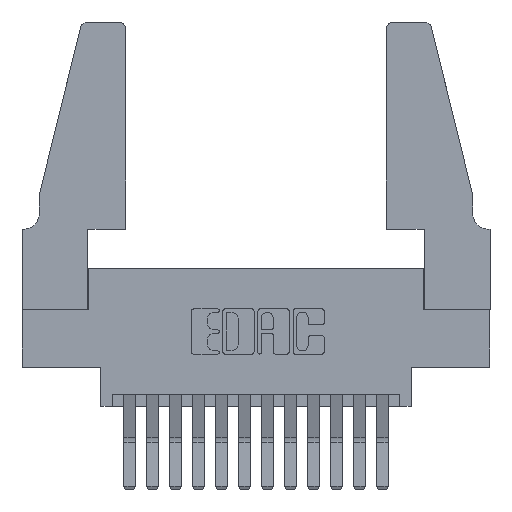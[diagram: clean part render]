
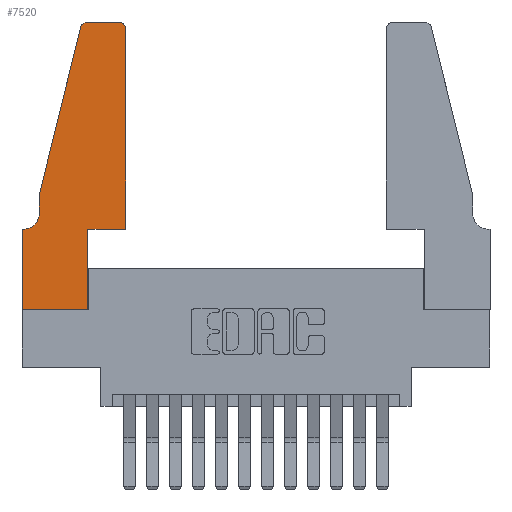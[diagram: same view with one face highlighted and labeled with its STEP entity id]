
A CAD part, top view. The second image highlights one B-rep face of the part: STEP entity #7520.
In plain terms, the highlighted planar face has unit normal (0, 0, 1).
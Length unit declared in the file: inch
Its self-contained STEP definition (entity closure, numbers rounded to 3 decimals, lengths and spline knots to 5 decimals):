
#479 = VECTOR ( 'NONE', #13768, 39.37008 ) ;
#505 = VERTEX_POINT ( 'NONE', #4299 ) ;
#840 = ORIENTED_EDGE ( 'NONE', *, *, #12736, .T. ) ;
#854 = ORIENTED_EDGE ( 'NONE', *, *, #15607, .T. ) ;
#908 = VERTEX_POINT ( 'NONE', #6339 ) ;
#961 = CARTESIAN_POINT ( 'NONE',  ( 0.0755, 0.35, 0.37 ) ) ;
#1022 = CIRCLE ( 'NONE', #14794, 0.07 ) ;
#1162 = CARTESIAN_POINT ( 'NONE',  ( 0.2865, 0.35, 0.37 ) ) ;
#1257 = VECTOR ( 'NONE', #4696, 39.37008 ) ;
#1304 = CARTESIAN_POINT ( 'NONE',  ( 0., 0., 0.37 ) ) ;
#1412 = ORIENTED_EDGE ( 'NONE', *, *, #11370, .T. ) ;
#1594 = CARTESIAN_POINT ( 'NONE',  ( 0.4505, 0.35, 0.37 ) ) ;
#1698 = EDGE_CURVE ( 'NONE', #505, #10028, #10328, .T. ) ;
#2288 = CARTESIAN_POINT ( 'NONE',  ( 0.4505, 0.35, 0.37 ) ) ;
#2584 = CARTESIAN_POINT ( 'NONE',  ( 0.4505, 0.35, 0.37 ) ) ;
#2768 = CARTESIAN_POINT ( 'NONE',  ( 0.0755, 0.5, 0.37 ) ) ;
#2805 = FACE_OUTER_BOUND ( 'NONE', #8059, .T. ) ;
#2942 = ORIENTED_EDGE ( 'NONE', *, *, #3870, .T. ) ;
#3148 = EDGE_CURVE ( 'NONE', #4799, #7429, #10499, .T. ) ;
#3247 = DIRECTION ( 'NONE',  ( 0., 1., 0. ) ) ;
#3351 = ORIENTED_EDGE ( 'NONE', *, *, #1698, .T. ) ;
#3458 = CIRCLE ( 'NONE', #11859, 0.03 ) ;
#3568 = LINE ( 'NONE', #2288, #15792 ) ;
#3857 = ORIENTED_EDGE ( 'NONE', *, *, #7246, .T. ) ;
#3870 = EDGE_CURVE ( 'NONE', #908, #11900, #13497, .T. ) ;
#4131 = LINE ( 'NONE', #1304, #12725 ) ;
#4299 = CARTESIAN_POINT ( 'NONE',  ( 0.0055, 0.35, 0.37 ) ) ;
#4397 = CARTESIAN_POINT ( 'NONE',  ( 0.0055, 0.42, 0.37 ) ) ;
#4409 = DIRECTION ( 'NONE',  ( -1., 0., 0. ) ) ;
#4422 = EDGE_CURVE ( 'NONE', #11900, #8486, #15194, .T. ) ;
#4696 = DIRECTION ( 'NONE',  ( -1., 0., 0. ) ) ;
#4799 = VERTEX_POINT ( 'NONE', #15461 ) ;
#4889 = PLANE ( 'NONE',  #12070 ) ;
#5091 = CARTESIAN_POINT ( 'NONE',  ( 0.284, 1.22, 0.37 ) ) ;
#5135 = DIRECTION ( 'NONE',  ( 0., 0., 1. ) ) ;
#5478 = ORIENTED_EDGE ( 'NONE', *, *, #8214, .T. ) ;
#5525 = CARTESIAN_POINT ( 'NONE',  ( 0.0755, 0.42, 0.37 ) ) ;
#5592 = CARTESIAN_POINT ( 'NONE',  ( 0.2605, 1.25, 0.37 ) ) ;
#5638 = DIRECTION ( 'NONE',  ( -1., 0., 0. ) ) ;
#5764 = CARTESIAN_POINT ( 'NONE',  ( 0.284, 1.25, 0.37 ) ) ;
#5766 = ORIENTED_EDGE ( 'NONE', *, *, #13067, .T. ) ;
#6056 = ORIENTED_EDGE ( 'NONE', *, *, #4422, .T. ) ;
#6155 = CARTESIAN_POINT ( 'NONE',  ( 0., 0.35, 0.37 ) ) ;
#6177 = LINE ( 'NONE', #13020, #12276 ) ;
#6339 = CARTESIAN_POINT ( 'NONE',  ( 0.25487, 1.22718, 0.37 ) ) ;
#6356 = DIRECTION ( 'NONE',  ( 1., 0., 0. ) ) ;
#7021 = AXIS2_PLACEMENT_3D ( 'NONE', #12463, #5135, #13675 ) ;
#7246 = EDGE_CURVE ( 'NONE', #8486, #505, #1022, .T. ) ;
#7361 = DIRECTION ( 'NONE',  ( 1., 0., 0. ) ) ;
#7429 = VERTEX_POINT ( 'NONE', #13243 ) ;
#7454 = DIRECTION ( 'NONE',  ( 1., 0., 0. ) ) ;
#7463 = DIRECTION ( 'NONE',  ( 0., -1., 0. ) ) ;
#7502 = VERTEX_POINT ( 'NONE', #1162 ) ;
#7520 = ADVANCED_FACE ( 'NONE', ( #2805 ), #4889, .T. ) ;
#7588 = VERTEX_POINT ( 'NONE', #11174 ) ;
#7688 = VERTEX_POINT ( 'NONE', #8889 ) ;
#7947 = LINE ( 'NONE', #5592, #10430 ) ;
#7971 = VERTEX_POINT ( 'NONE', #5764 ) ;
#8059 = EDGE_LOOP ( 'NONE', ( #5766, #854, #2942, #6056, #3857, #3351, #14340, #5478, #15771, #1412, #840, #13711 ) ) ;
#8214 = EDGE_CURVE ( 'NONE', #7588, #7688, #4131, .T. ) ;
#8486 = VERTEX_POINT ( 'NONE', #5525 ) ;
#8522 = CARTESIAN_POINT ( 'NONE',  ( 0., 0., 0.37 ) ) ;
#8798 = EDGE_CURVE ( 'NONE', #10028, #7588, #15186, .T. ) ;
#8889 = CARTESIAN_POINT ( 'NONE',  ( 0.2865, 0., 0.37 ) ) ;
#9663 = LINE ( 'NONE', #2584, #12133 ) ;
#10028 = VERTEX_POINT ( 'NONE', #11047 ) ;
#10328 = LINE ( 'NONE', #961, #1257 ) ;
#10430 = VECTOR ( 'NONE', #4409, 39.37008 ) ;
#10499 = CIRCLE ( 'NONE', #7021, 0.03 ) ;
#10548 = EDGE_CURVE ( 'NONE', #7688, #7502, #6177, .T. ) ;
#10970 = DIRECTION ( 'NONE',  ( 0., -1., 0. ) ) ;
#10986 = VERTEX_POINT ( 'NONE', #1594 ) ;
#11047 = CARTESIAN_POINT ( 'NONE',  ( 0., 0.35, 0.37 ) ) ;
#11174 = CARTESIAN_POINT ( 'NONE',  ( 0., 0., 0.37 ) ) ;
#11370 = EDGE_CURVE ( 'NONE', #7502, #10986, #3568, .T. ) ;
#11859 = AXIS2_PLACEMENT_3D ( 'NONE', #5091, #13640, #6356 ) ;
#11900 = VERTEX_POINT ( 'NONE', #13078 ) ;
#11961 = VECTOR ( 'NONE', #7463, 39.37008 ) ;
#12070 = AXIS2_PLACEMENT_3D ( 'NONE', #6155, #14636, #7361 ) ;
#12133 = VECTOR ( 'NONE', #14737, 39.37008 ) ;
#12276 = VECTOR ( 'NONE', #3247, 39.37008 ) ;
#12321 = CARTESIAN_POINT ( 'NONE',  ( 0.0755, 0.5, 0.37 ) ) ;
#12463 = CARTESIAN_POINT ( 'NONE',  ( 0.4205, 1.22, 0.37 ) ) ;
#12725 = VECTOR ( 'NONE', #7454, 39.37008 ) ;
#12736 = EDGE_CURVE ( 'NONE', #10986, #4799, #9663, .T. ) ;
#12936 = DIRECTION ( 'NONE',  ( 0., 0., -1. ) ) ;
#13020 = CARTESIAN_POINT ( 'NONE',  ( 0.2865, 0.35, 0.37 ) ) ;
#13067 = EDGE_CURVE ( 'NONE', #7429, #7971, #7947, .T. ) ;
#13078 = CARTESIAN_POINT ( 'NONE',  ( 0.0755, 0.5, 0.37 ) ) ;
#13243 = CARTESIAN_POINT ( 'NONE',  ( 0.4205, 1.25, 0.37 ) ) ;
#13298 = DIRECTION ( 'NONE',  ( 1., 0., 0. ) ) ;
#13497 = LINE ( 'NONE', #2768, #479 ) ;
#13640 = DIRECTION ( 'NONE',  ( 0., 0., 1. ) ) ;
#13675 = DIRECTION ( 'NONE',  ( 1., 0., 0. ) ) ;
#13711 = ORIENTED_EDGE ( 'NONE', *, *, #3148, .T. ) ;
#13768 = DIRECTION ( 'NONE',  ( -0.239, -0.971, 0. ) ) ;
#14340 = ORIENTED_EDGE ( 'NONE', *, *, #8798, .T. ) ;
#14391 = VECTOR ( 'NONE', #10970, 39.37008 ) ;
#14636 = DIRECTION ( 'NONE',  ( 0., 0., 1. ) ) ;
#14737 = DIRECTION ( 'NONE',  ( 0., 1., 0. ) ) ;
#14794 = AXIS2_PLACEMENT_3D ( 'NONE', #4397, #12936, #5638 ) ;
#15186 = LINE ( 'NONE', #8522, #14391 ) ;
#15194 = LINE ( 'NONE', #12321, #11961 ) ;
#15461 = CARTESIAN_POINT ( 'NONE',  ( 0.4505, 1.22, 0.37 ) ) ;
#15607 = EDGE_CURVE ( 'NONE', #7971, #908, #3458, .T. ) ;
#15771 = ORIENTED_EDGE ( 'NONE', *, *, #10548, .T. ) ;
#15792 = VECTOR ( 'NONE', #13298, 39.37008 ) ;
